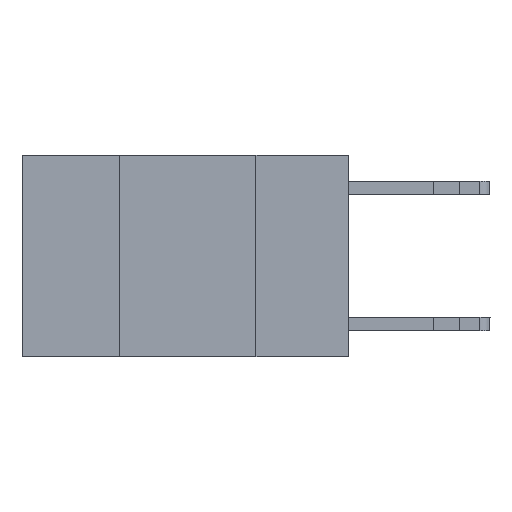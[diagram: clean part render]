
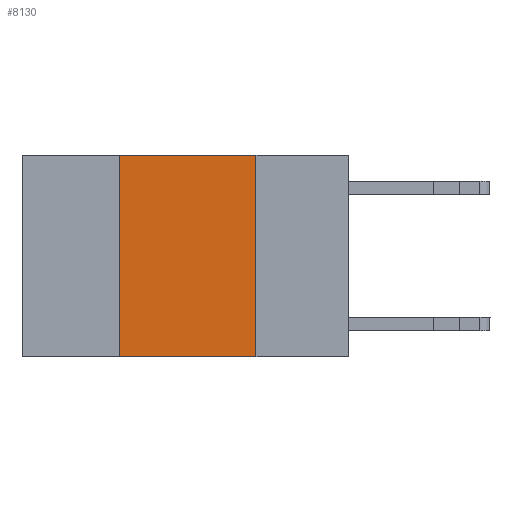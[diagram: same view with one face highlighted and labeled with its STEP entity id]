
A CAD part, left-side view. The second image highlights one B-rep face of the part: STEP entity #8130.
In plain terms, the highlighted planar face has unit normal (-1, 0, 0).
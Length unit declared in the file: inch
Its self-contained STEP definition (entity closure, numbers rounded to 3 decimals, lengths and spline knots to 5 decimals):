
#258 = ORIENTED_EDGE ( 'NONE', *, *, #12944, .F. ) ;
#1300 = EDGE_CURVE ( 'NONE', #19671, #4241, #13514, .T. ) ;
#1443 = CARTESIAN_POINT ( 'NONE',  ( 0., 0.6, 0. ) ) ;
#3581 = CARTESIAN_POINT ( 'NONE',  ( 0., 0.42, 0. ) ) ;
#4241 = VERTEX_POINT ( 'NONE', #14328 ) ;
#4313 = LINE ( 'NONE', #3581, #12147 ) ;
#5313 = VECTOR ( 'NONE', #14541, 39.37008 ) ;
#8130 = ADVANCED_FACE ( 'NONE', ( #12014 ), #14255, .F. ) ;
#8158 = CARTESIAN_POINT ( 'NONE',  ( 0., 0.6, 0. ) ) ;
#8339 = DIRECTION ( 'NONE',  ( 0., 0., 1. ) ) ;
#8360 = CARTESIAN_POINT ( 'NONE',  ( 0., 0.17, -0.37 ) ) ;
#8962 = VECTOR ( 'NONE', #12688, 39.37008 ) ;
#9255 = CARTESIAN_POINT ( 'NONE',  ( 0., 0.42, 0. ) ) ;
#9495 = LINE ( 'NONE', #13039, #5313 ) ;
#9733 = DIRECTION ( 'NONE',  ( 0., 0., -1. ) ) ;
#10249 = VERTEX_POINT ( 'NONE', #8360 ) ;
#10887 = EDGE_CURVE ( 'NONE', #16275, #19671, #4313, .T. ) ;
#11791 = ORIENTED_EDGE ( 'NONE', *, *, #19303, .T. ) ;
#12014 = FACE_OUTER_BOUND ( 'NONE', #18150, .T. ) ;
#12147 = VECTOR ( 'NONE', #8339, 39.37008 ) ;
#12688 = DIRECTION ( 'NONE',  ( 0., -1., 0. ) ) ;
#12944 = EDGE_CURVE ( 'NONE', #4241, #10249, #17034, .T. ) ;
#13039 = CARTESIAN_POINT ( 'NONE',  ( 0., 0.6, -0.37 ) ) ;
#13514 = LINE ( 'NONE', #1443, #8962 ) ;
#14255 = PLANE ( 'NONE',  #15880 ) ;
#14291 = DIRECTION ( 'NONE',  ( 0., 0., -1. ) ) ;
#14328 = CARTESIAN_POINT ( 'NONE',  ( 0., 0.17, 0. ) ) ;
#14356 = CARTESIAN_POINT ( 'NONE',  ( 0., 0.17, 0. ) ) ;
#14541 = DIRECTION ( 'NONE',  ( 0., -1., 0. ) ) ;
#15880 = AXIS2_PLACEMENT_3D ( 'NONE', #8158, #18757, #9733 ) ;
#16246 = ORIENTED_EDGE ( 'NONE', *, *, #1300, .F. ) ;
#16275 = VERTEX_POINT ( 'NONE', #19051 ) ;
#16545 = VECTOR ( 'NONE', #14291, 39.37008 ) ;
#17034 = LINE ( 'NONE', #14356, #16545 ) ;
#18150 = EDGE_LOOP ( 'NONE', ( #258, #16246, #19707, #11791 ) ) ;
#18757 = DIRECTION ( 'NONE',  ( 1., 0., 0. ) ) ;
#19051 = CARTESIAN_POINT ( 'NONE',  ( 0., 0.42, -0.37 ) ) ;
#19303 = EDGE_CURVE ( 'NONE', #16275, #10249, #9495, .T. ) ;
#19671 = VERTEX_POINT ( 'NONE', #9255 ) ;
#19707 = ORIENTED_EDGE ( 'NONE', *, *, #10887, .F. ) ;
